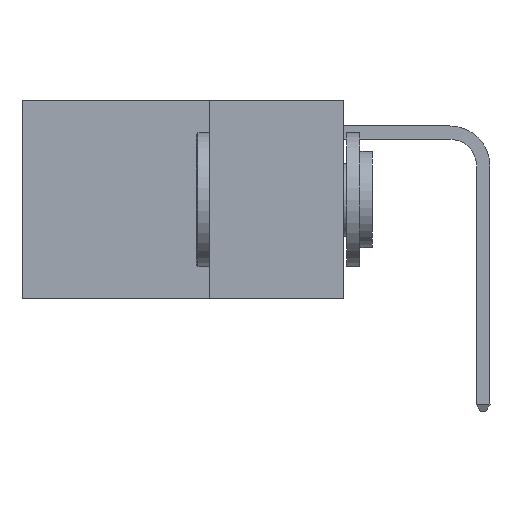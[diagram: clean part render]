
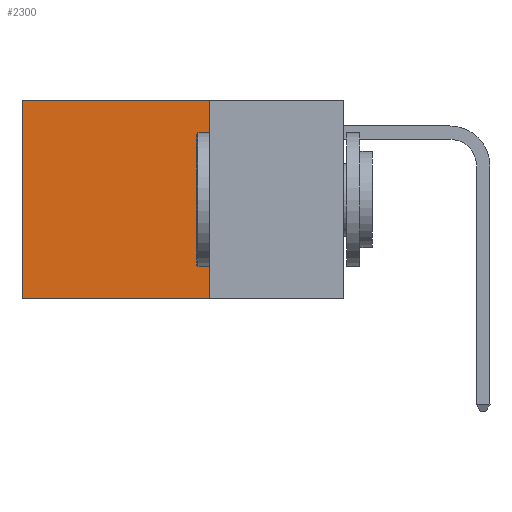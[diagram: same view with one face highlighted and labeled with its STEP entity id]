
A CAD part, left-side view. The second image highlights one B-rep face of the part: STEP entity #2300.
In plain terms, the highlighted planar face has unit normal (-1, 0, 0).
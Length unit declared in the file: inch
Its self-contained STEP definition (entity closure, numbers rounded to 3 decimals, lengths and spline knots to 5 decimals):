
#162 = DIRECTION ( 'NONE',  ( 0., 0., -1. ) ) ;
#187 = CARTESIAN_POINT ( 'NONE',  ( 0.2625, 0.6, 0. ) ) ;
#485 = CARTESIAN_POINT ( 'NONE',  ( 0.2625, 0.25, 0. ) ) ;
#899 = DIRECTION ( 'NONE',  ( 0., 1., 0. ) ) ;
#986 = CARTESIAN_POINT ( 'NONE',  ( 0.2625, 0.25, 0. ) ) ;
#1102 = CARTESIAN_POINT ( 'NONE',  ( 0.2625, 0.6, -0.37 ) ) ;
#2138 = VECTOR ( 'NONE', #4520, 39.37008 ) ;
#2193 = CARTESIAN_POINT ( 'NONE',  ( 0.2625, 0.6, 0. ) ) ;
#2300 = ADVANCED_FACE ( 'NONE', ( #9216 ), #5936, .F. ) ;
#2317 = LINE ( 'NONE', #6697, #2138 ) ;
#4321 = CARTESIAN_POINT ( 'NONE',  ( 0.2625, 0.25, 0. ) ) ;
#4353 = AXIS2_PLACEMENT_3D ( 'NONE', #6133, #5925, #5910 ) ;
#4520 = DIRECTION ( 'NONE',  ( 0., 1., 0. ) ) ;
#5060 = VERTEX_POINT ( 'NONE', #2193 ) ;
#5336 = VERTEX_POINT ( 'NONE', #986 ) ;
#5681 = VERTEX_POINT ( 'NONE', #1102 ) ;
#5846 = VERTEX_POINT ( 'NONE', #10850 ) ;
#5910 = DIRECTION ( 'NONE',  ( 0., 0., -1. ) ) ;
#5925 = DIRECTION ( 'NONE',  ( 1., 0., 0. ) ) ;
#5936 = PLANE ( 'NONE',  #4353 ) ;
#6133 = CARTESIAN_POINT ( 'NONE',  ( 0.2625, 0.25, 0. ) ) ;
#6514 = EDGE_LOOP ( 'NONE', ( #10170, #11911, #8710, #7173 ) ) ;
#6547 = LINE ( 'NONE', #485, #9814 ) ;
#6697 = CARTESIAN_POINT ( 'NONE',  ( 0.2625, 0.25, -0.37 ) ) ;
#6779 = EDGE_CURVE ( 'NONE', #5336, #5060, #11623, .T. ) ;
#7001 = EDGE_CURVE ( 'NONE', #5060, #5681, #10287, .T. ) ;
#7173 = ORIENTED_EDGE ( 'NONE', *, *, #6779, .T. ) ;
#8710 = ORIENTED_EDGE ( 'NONE', *, *, #12285, .F. ) ;
#9216 = FACE_OUTER_BOUND ( 'NONE', #6514, .T. ) ;
#9463 = EDGE_CURVE ( 'NONE', #5846, #5681, #2317, .T. ) ;
#9814 = VECTOR ( 'NONE', #162, 39.37008 ) ;
#10170 = ORIENTED_EDGE ( 'NONE', *, *, #7001, .T. ) ;
#10247 = VECTOR ( 'NONE', #12140, 39.37008 ) ;
#10287 = LINE ( 'NONE', #187, #10247 ) ;
#10850 = CARTESIAN_POINT ( 'NONE',  ( 0.2625, 0.25, -0.37 ) ) ;
#11570 = VECTOR ( 'NONE', #899, 39.37008 ) ;
#11623 = LINE ( 'NONE', #4321, #11570 ) ;
#11911 = ORIENTED_EDGE ( 'NONE', *, *, #9463, .F. ) ;
#12140 = DIRECTION ( 'NONE',  ( 0., 0., -1. ) ) ;
#12285 = EDGE_CURVE ( 'NONE', #5336, #5846, #6547, .T. ) ;
